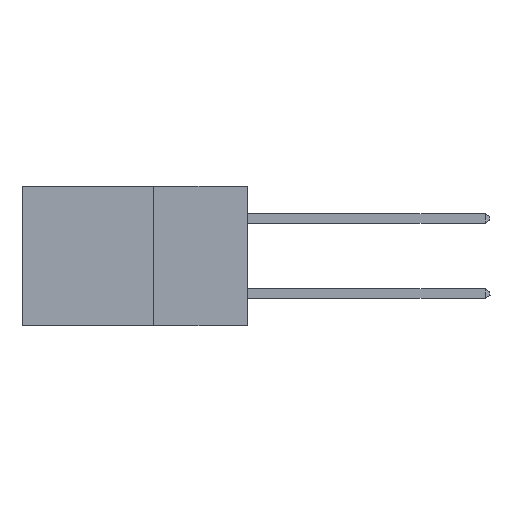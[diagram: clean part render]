
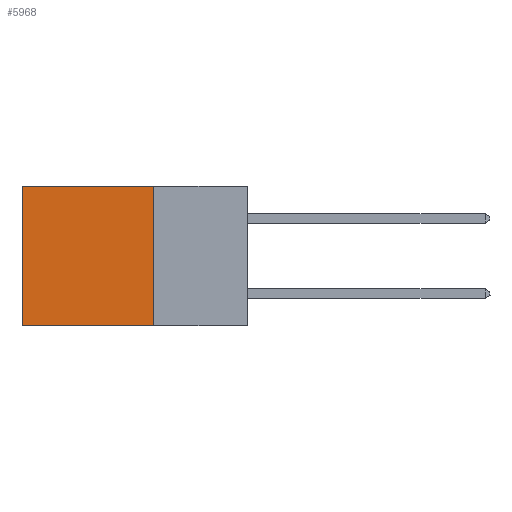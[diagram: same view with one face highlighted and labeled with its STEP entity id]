
A CAD part, left-side view. The second image highlights one B-rep face of the part: STEP entity #5968.
In plain terms, the highlighted planar face has unit normal (-1, 0, 0).
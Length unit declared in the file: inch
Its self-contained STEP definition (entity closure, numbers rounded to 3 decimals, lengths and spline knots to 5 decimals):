
#777 = EDGE_CURVE ( 'NONE', #11444, #6166, #1045, .T. ) ;
#1045 = LINE ( 'NONE', #1259, #11520 ) ;
#1049 = EDGE_CURVE ( 'NONE', #6166, #9403, #12604, .T. ) ;
#1130 = PLANE ( 'NONE',  #3867 ) ;
#1259 = CARTESIAN_POINT ( 'NONE',  ( 0.298, 0.25, 0. ) ) ;
#1560 = VECTOR ( 'NONE', #14559, 39.37008 ) ;
#1761 = VECTOR ( 'NONE', #22273, 39.37008 ) ;
#2207 = LINE ( 'NONE', #7623, #3835 ) ;
#2285 = VERTEX_POINT ( 'NONE', #19978 ) ;
#3835 = VECTOR ( 'NONE', #20021, 39.37008 ) ;
#3867 = AXIS2_PLACEMENT_3D ( 'NONE', #8444, #15203, #16897 ) ;
#5340 = ORIENTED_EDGE ( 'NONE', *, *, #16022, .F. ) ;
#5968 = ADVANCED_FACE ( 'NONE', ( #20052 ), #1130, .F. ) ;
#6166 = VERTEX_POINT ( 'NONE', #10288 ) ;
#6259 = CARTESIAN_POINT ( 'NONE',  ( 0.298, 0.25, -0.37 ) ) ;
#7246 = ORIENTED_EDGE ( 'NONE', *, *, #777, .T. ) ;
#7400 = CARTESIAN_POINT ( 'NONE',  ( 0.298, 0.6, 0. ) ) ;
#7623 = CARTESIAN_POINT ( 'NONE',  ( 0.298, 0.25, 0. ) ) ;
#8100 = LINE ( 'NONE', #6259, #1761 ) ;
#8444 = CARTESIAN_POINT ( 'NONE',  ( 0.298, 0.25, 0. ) ) ;
#9403 = VERTEX_POINT ( 'NONE', #11741 ) ;
#9602 = CARTESIAN_POINT ( 'NONE',  ( 0.298, 0.25, 0. ) ) ;
#10288 = CARTESIAN_POINT ( 'NONE',  ( 0.298, 0.6, 0. ) ) ;
#11444 = VERTEX_POINT ( 'NONE', #9602 ) ;
#11520 = VECTOR ( 'NONE', #12041, 39.37008 ) ;
#11741 = CARTESIAN_POINT ( 'NONE',  ( 0.298, 0.6, -0.37 ) ) ;
#12041 = DIRECTION ( 'NONE',  ( 0., 1., 0. ) ) ;
#12604 = LINE ( 'NONE', #7400, #1560 ) ;
#14559 = DIRECTION ( 'NONE',  ( 0., 0., -1. ) ) ;
#15203 = DIRECTION ( 'NONE',  ( 1., 0., 0. ) ) ;
#16022 = EDGE_CURVE ( 'NONE', #2285, #9403, #8100, .T. ) ;
#16897 = DIRECTION ( 'NONE',  ( 0., 0., -1. ) ) ;
#19027 = EDGE_CURVE ( 'NONE', #11444, #2285, #2207, .T. ) ;
#19544 = EDGE_LOOP ( 'NONE', ( #21812, #5340, #19764, #7246 ) ) ;
#19764 = ORIENTED_EDGE ( 'NONE', *, *, #19027, .F. ) ;
#19978 = CARTESIAN_POINT ( 'NONE',  ( 0.298, 0.25, -0.37 ) ) ;
#20021 = DIRECTION ( 'NONE',  ( 0., 0., -1. ) ) ;
#20052 = FACE_OUTER_BOUND ( 'NONE', #19544, .T. ) ;
#21812 = ORIENTED_EDGE ( 'NONE', *, *, #1049, .T. ) ;
#22273 = DIRECTION ( 'NONE',  ( 0., 1., 0. ) ) ;
